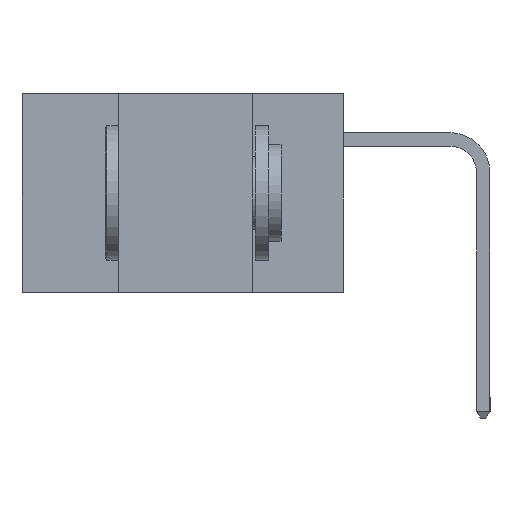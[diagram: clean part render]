
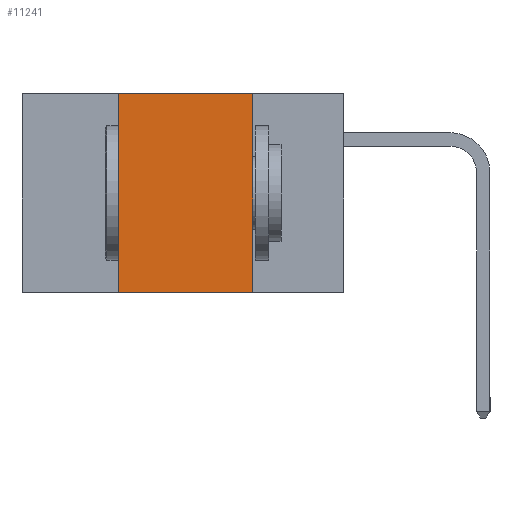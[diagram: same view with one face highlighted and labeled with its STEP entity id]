
A CAD part, left-side view. The second image highlights one B-rep face of the part: STEP entity #11241.
In plain terms, the highlighted planar face has unit normal (-1, 0, 0).
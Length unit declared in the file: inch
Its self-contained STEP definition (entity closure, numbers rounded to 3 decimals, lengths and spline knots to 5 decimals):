
#935 = PLANE ( 'NONE',  #1408 ) ;
#1131 = CARTESIAN_POINT ( 'NONE',  ( 0., 0.17, -0.37 ) ) ;
#1408 = AXIS2_PLACEMENT_3D ( 'NONE', #12704, #2537, #14340 ) ;
#1463 = DIRECTION ( 'NONE',  ( 0., 0., -1. ) ) ;
#1695 = CARTESIAN_POINT ( 'NONE',  ( 0., 0.17, -0.37 ) ) ;
#1893 = DIRECTION ( 'NONE',  ( 0., 0., 1. ) ) ;
#1954 = ORIENTED_EDGE ( 'NONE', *, *, #5260, .T. ) ;
#2512 = EDGE_CURVE ( 'NONE', #17018, #6724, #17606, .T. ) ;
#2537 = DIRECTION ( 'NONE',  ( 1., 0., 0. ) ) ;
#3587 = VECTOR ( 'NONE', #1893, 39.37008 ) ;
#5082 = LINE ( 'NONE', #11150, #13005 ) ;
#5260 = EDGE_CURVE ( 'NONE', #11688, #6724, #5082, .T. ) ;
#6252 = VERTEX_POINT ( 'NONE', #10674 ) ;
#6724 = VERTEX_POINT ( 'NONE', #1695 ) ;
#6891 = CARTESIAN_POINT ( 'NONE',  ( 0., 0.6, 0. ) ) ;
#8687 = EDGE_CURVE ( 'NONE', #11688, #6252, #9197, .T. ) ;
#9197 = LINE ( 'NONE', #15304, #3587 ) ;
#9963 = ORIENTED_EDGE ( 'NONE', *, *, #10928, .F. ) ;
#10056 = CARTESIAN_POINT ( 'NONE',  ( 0., 0.17, 0. ) ) ;
#10674 = CARTESIAN_POINT ( 'NONE',  ( 0., 0.42, 0. ) ) ;
#10928 = EDGE_CURVE ( 'NONE', #6252, #17018, #19971, .T. ) ;
#11150 = CARTESIAN_POINT ( 'NONE',  ( 0., 0.6, -0.37 ) ) ;
#11241 = ADVANCED_FACE ( 'NONE', ( #17758 ), #935, .F. ) ;
#11272 = DIRECTION ( 'NONE',  ( 0., -1., 0. ) ) ;
#11688 = VERTEX_POINT ( 'NONE', #15294 ) ;
#12704 = CARTESIAN_POINT ( 'NONE',  ( 0., 0.6, 0. ) ) ;
#13005 = VECTOR ( 'NONE', #11272, 39.37008 ) ;
#14340 = DIRECTION ( 'NONE',  ( 0., 0., -1. ) ) ;
#15267 = VECTOR ( 'NONE', #16813, 39.37008 ) ;
#15294 = CARTESIAN_POINT ( 'NONE',  ( 0., 0.42, -0.37 ) ) ;
#15304 = CARTESIAN_POINT ( 'NONE',  ( 0., 0.42, -0.37 ) ) ;
#16813 = DIRECTION ( 'NONE',  ( 0., -1., 0. ) ) ;
#17018 = VERTEX_POINT ( 'NONE', #10056 ) ;
#17106 = VECTOR ( 'NONE', #1463, 39.37008 ) ;
#17606 = LINE ( 'NONE', #1131, #17106 ) ;
#17758 = FACE_OUTER_BOUND ( 'NONE', #18871, .T. ) ;
#18544 = ORIENTED_EDGE ( 'NONE', *, *, #8687, .F. ) ;
#18871 = EDGE_LOOP ( 'NONE', ( #20761, #9963, #18544, #1954 ) ) ;
#19971 = LINE ( 'NONE', #6891, #15267 ) ;
#20761 = ORIENTED_EDGE ( 'NONE', *, *, #2512, .F. ) ;
